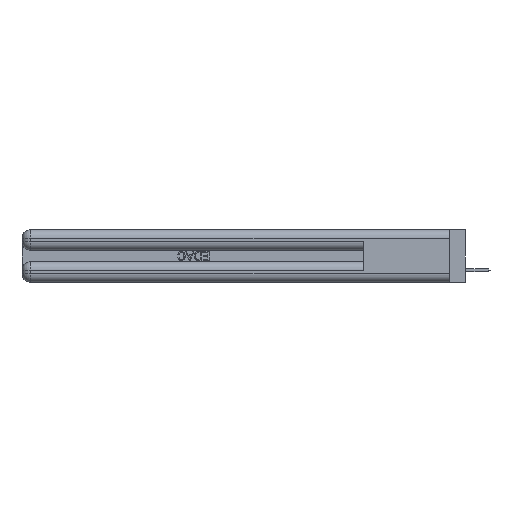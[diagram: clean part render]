
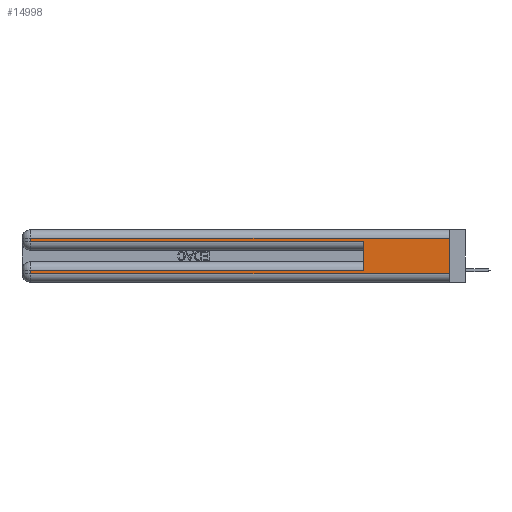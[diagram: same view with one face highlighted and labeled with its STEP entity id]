
A CAD part, left-side view. The second image highlights one B-rep face of the part: STEP entity #14998.
In plain terms, the highlighted planar face has unit normal (-1, 0, 0).
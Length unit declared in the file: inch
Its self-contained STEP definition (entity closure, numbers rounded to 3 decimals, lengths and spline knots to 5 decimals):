
#90 = FACE_OUTER_BOUND ( 'NONE', #12141, .T. ) ;
#390 = VERTEX_POINT ( 'NONE', #29811 ) ;
#860 = VERTEX_POINT ( 'NONE', #20359 ) ;
#1517 = CARTESIAN_POINT ( 'NONE',  ( 0., 0., 0.085 ) ) ;
#2149 = LINE ( 'NONE', #16031, #42348 ) ;
#2946 = VECTOR ( 'NONE', #19489, 39.37008 ) ;
#3531 = VECTOR ( 'NONE', #21989, 39.37008 ) ;
#4141 = EDGE_CURVE ( 'NONE', #17359, #390, #39309, .T. ) ;
#5383 = DIRECTION ( 'NONE',  ( 0., 1., 0. ) ) ;
#5408 = EDGE_CURVE ( 'NONE', #39019, #860, #15980, .T. ) ;
#5816 = CARTESIAN_POINT ( 'NONE',  ( 0., 0., 0.06 ) ) ;
#7285 = ORIENTED_EDGE ( 'NONE', *, *, #4141, .T. ) ;
#7460 = EDGE_CURVE ( 'NONE', #17359, #28587, #21388, .T. ) ;
#7502 = CARTESIAN_POINT ( 'NONE',  ( 0., 2.94, 0.06 ) ) ;
#8722 = CARTESIAN_POINT ( 'NONE',  ( 0., 0., 0.37 ) ) ;
#9030 = AXIS2_PLACEMENT_3D ( 'NONE', #8722, #12092, #18441 ) ;
#10548 = CARTESIAN_POINT ( 'NONE',  ( 0., 2.94, 0.085 ) ) ;
#11180 = DIRECTION ( 'NONE',  ( 0., 1., 0. ) ) ;
#12092 = DIRECTION ( 'NONE',  ( 1., 0., 0. ) ) ;
#12141 = EDGE_LOOP ( 'NONE', ( #32856, #7285, #30801, #30630, #26557, #13556, #15008, #19256 ) ) ;
#12233 = EDGE_CURVE ( 'NONE', #390, #26954, #30651, .T. ) ;
#13556 = ORIENTED_EDGE ( 'NONE', *, *, #25618, .T. ) ;
#14886 = DIRECTION ( 'NONE',  ( 0., 0., 1. ) ) ;
#14998 = ADVANCED_FACE ( 'NONE', ( #90 ), #28764, .F. ) ;
#15008 = ORIENTED_EDGE ( 'NONE', *, *, #42961, .T. ) ;
#15684 = EDGE_CURVE ( 'NONE', #26954, #860, #27282, .T. ) ;
#15689 = VECTOR ( 'NONE', #5383, 39.37008 ) ;
#15872 = CARTESIAN_POINT ( 'NONE',  ( 0., 2.94, 0.285 ) ) ;
#15980 = LINE ( 'NONE', #38228, #39437 ) ;
#16031 = CARTESIAN_POINT ( 'NONE',  ( 0., 2.94, 0.37 ) ) ;
#17359 = VERTEX_POINT ( 'NONE', #21675 ) ;
#18441 = DIRECTION ( 'NONE',  ( 0., 0., -1. ) ) ;
#18477 = VECTOR ( 'NONE', #11180, 39.37008 ) ;
#19256 = ORIENTED_EDGE ( 'NONE', *, *, #20286, .T. ) ;
#19489 = DIRECTION ( 'NONE',  ( 0., 0., -1. ) ) ;
#19899 = VECTOR ( 'NONE', #43155, 39.37008 ) ;
#20286 = EDGE_CURVE ( 'NONE', #30681, #28587, #32458, .T. ) ;
#20359 = CARTESIAN_POINT ( 'NONE',  ( 0., 0.6, 0.285 ) ) ;
#21388 = LINE ( 'NONE', #35346, #3531 ) ;
#21675 = CARTESIAN_POINT ( 'NONE',  ( 0., 0., 0.31 ) ) ;
#21989 = DIRECTION ( 'NONE',  ( 0., 0., -1. ) ) ;
#25618 = EDGE_CURVE ( 'NONE', #39019, #40783, #40788, .T. ) ;
#26557 = ORIENTED_EDGE ( 'NONE', *, *, #5408, .F. ) ;
#26954 = VERTEX_POINT ( 'NONE', #15872 ) ;
#27282 = LINE ( 'NONE', #30073, #19899 ) ;
#27333 = CARTESIAN_POINT ( 'NONE',  ( 0., 0.6, 0.085 ) ) ;
#28587 = VERTEX_POINT ( 'NONE', #5816 ) ;
#28764 = PLANE ( 'NONE',  #9030 ) ;
#29811 = CARTESIAN_POINT ( 'NONE',  ( 0., 2.94, 0.31 ) ) ;
#30073 = CARTESIAN_POINT ( 'NONE',  ( 0., 0., 0.285 ) ) ;
#30630 = ORIENTED_EDGE ( 'NONE', *, *, #15684, .T. ) ;
#30651 = LINE ( 'NONE', #42188, #2946 ) ;
#30681 = VERTEX_POINT ( 'NONE', #7502 ) ;
#30801 = ORIENTED_EDGE ( 'NONE', *, *, #12233, .T. ) ;
#31449 = CARTESIAN_POINT ( 'NONE',  ( 0., 0., 0.31 ) ) ;
#32458 = LINE ( 'NONE', #34661, #40290 ) ;
#32856 = ORIENTED_EDGE ( 'NONE', *, *, #7460, .F. ) ;
#34661 = CARTESIAN_POINT ( 'NONE',  ( 0., 0., 0.06 ) ) ;
#35346 = CARTESIAN_POINT ( 'NONE',  ( 0., 0., 0.37 ) ) ;
#38019 = DIRECTION ( 'NONE',  ( 0., -1., 0. ) ) ;
#38228 = CARTESIAN_POINT ( 'NONE',  ( 0., 0.6, 0.145 ) ) ;
#39019 = VERTEX_POINT ( 'NONE', #27333 ) ;
#39309 = LINE ( 'NONE', #31449, #18477 ) ;
#39349 = DIRECTION ( 'NONE',  ( 0., 0., -1. ) ) ;
#39437 = VECTOR ( 'NONE', #14886, 39.37008 ) ;
#40290 = VECTOR ( 'NONE', #38019, 39.37008 ) ;
#40783 = VERTEX_POINT ( 'NONE', #10548 ) ;
#40788 = LINE ( 'NONE', #1517, #15689 ) ;
#42188 = CARTESIAN_POINT ( 'NONE',  ( 0., 2.94, 0.37 ) ) ;
#42348 = VECTOR ( 'NONE', #39349, 39.37008 ) ;
#42961 = EDGE_CURVE ( 'NONE', #40783, #30681, #2149, .T. ) ;
#43155 = DIRECTION ( 'NONE',  ( 0., -1., 0. ) ) ;
